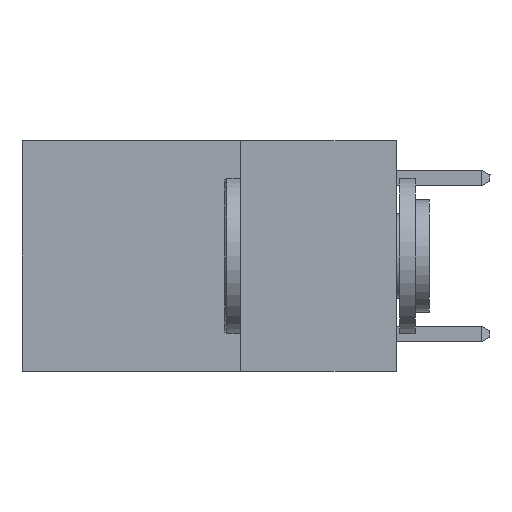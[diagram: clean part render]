
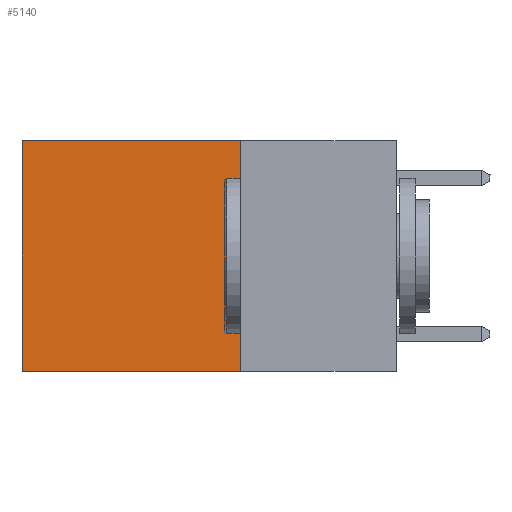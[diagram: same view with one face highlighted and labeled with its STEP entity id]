
A CAD part, left-side view. The second image highlights one B-rep face of the part: STEP entity #5140.
In plain terms, the highlighted planar face has unit normal (-1, 0, 0).
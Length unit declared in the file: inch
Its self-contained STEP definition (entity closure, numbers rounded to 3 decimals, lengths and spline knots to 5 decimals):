
#95 = CARTESIAN_POINT ( 'NONE',  ( 0.2625, 0.6, -0.37 ) ) ;
#156 = LINE ( 'NONE', #3842, #13753 ) ;
#352 = EDGE_LOOP ( 'NONE', ( #11105, #3614, #3470, #15443 ) ) ;
#737 = CARTESIAN_POINT ( 'NONE',  ( 0.2625, 0.25, 0. ) ) ;
#923 = CARTESIAN_POINT ( 'NONE',  ( 0.2625, 0.25, 0. ) ) ;
#1013 = DIRECTION ( 'NONE',  ( 0., 0., -1. ) ) ;
#3368 = VECTOR ( 'NONE', #9577, 39.37008 ) ;
#3470 = ORIENTED_EDGE ( 'NONE', *, *, #3700, .F. ) ;
#3614 = ORIENTED_EDGE ( 'NONE', *, *, #6485, .F. ) ;
#3700 = EDGE_CURVE ( 'NONE', #5358, #9653, #6766, .T. ) ;
#3842 = CARTESIAN_POINT ( 'NONE',  ( 0.2625, 0.6, 0. ) ) ;
#4229 = EDGE_CURVE ( 'NONE', #5358, #6526, #12377, .T. ) ;
#4979 = CARTESIAN_POINT ( 'NONE',  ( 0.2625, 0.25, 0. ) ) ;
#5140 = ADVANCED_FACE ( 'NONE', ( #11930 ), #12091, .F. ) ;
#5174 = DIRECTION ( 'NONE',  ( 0., 1., 0. ) ) ;
#5358 = VERTEX_POINT ( 'NONE', #14404 ) ;
#5912 = DIRECTION ( 'NONE',  ( 1., 0., 0. ) ) ;
#6309 = CARTESIAN_POINT ( 'NONE',  ( 0.2625, 0.6, 0. ) ) ;
#6485 = EDGE_CURVE ( 'NONE', #9653, #11247, #7539, .T. ) ;
#6526 = VERTEX_POINT ( 'NONE', #6309 ) ;
#6766 = LINE ( 'NONE', #737, #3368 ) ;
#7539 = LINE ( 'NONE', #12510, #15403 ) ;
#9130 = VECTOR ( 'NONE', #15789, 39.37008 ) ;
#9577 = DIRECTION ( 'NONE',  ( 0., 0., -1. ) ) ;
#9653 = VERTEX_POINT ( 'NONE', #15812 ) ;
#11105 = ORIENTED_EDGE ( 'NONE', *, *, #13155, .T. ) ;
#11247 = VERTEX_POINT ( 'NONE', #95 ) ;
#11930 = FACE_OUTER_BOUND ( 'NONE', #352, .T. ) ;
#12091 = PLANE ( 'NONE',  #15628 ) ;
#12377 = LINE ( 'NONE', #4979, #9130 ) ;
#12510 = CARTESIAN_POINT ( 'NONE',  ( 0.2625, 0.25, -0.37 ) ) ;
#13155 = EDGE_CURVE ( 'NONE', #6526, #11247, #156, .T. ) ;
#13753 = VECTOR ( 'NONE', #14892, 39.37008 ) ;
#14404 = CARTESIAN_POINT ( 'NONE',  ( 0.2625, 0.25, 0. ) ) ;
#14892 = DIRECTION ( 'NONE',  ( 0., 0., -1. ) ) ;
#15403 = VECTOR ( 'NONE', #5174, 39.37008 ) ;
#15443 = ORIENTED_EDGE ( 'NONE', *, *, #4229, .T. ) ;
#15628 = AXIS2_PLACEMENT_3D ( 'NONE', #923, #5912, #1013 ) ;
#15789 = DIRECTION ( 'NONE',  ( 0., 1., 0. ) ) ;
#15812 = CARTESIAN_POINT ( 'NONE',  ( 0.2625, 0.25, -0.37 ) ) ;
